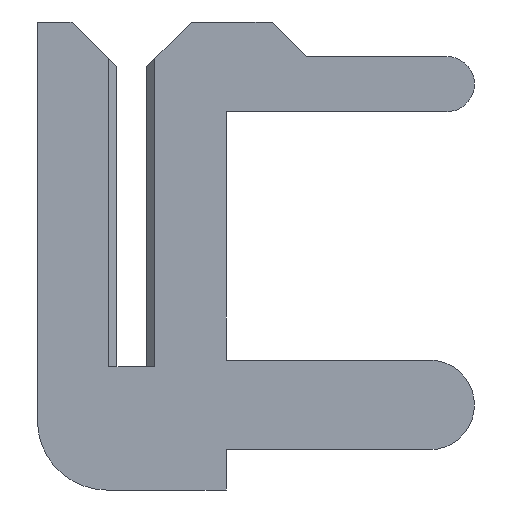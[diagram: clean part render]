
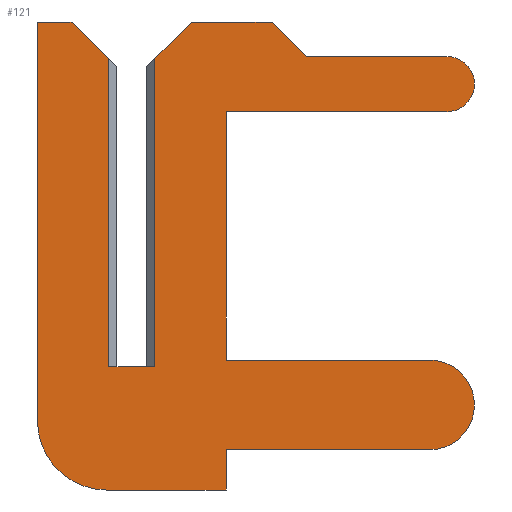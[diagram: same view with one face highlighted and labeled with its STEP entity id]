
A CAD part, left-side view. The second image highlights one B-rep face of the part: STEP entity #121.
In plain terms, the highlighted planar face has unit normal (-1, 0, 0).
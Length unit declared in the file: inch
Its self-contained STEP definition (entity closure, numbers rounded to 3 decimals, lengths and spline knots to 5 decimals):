
#1 = CARTESIAN_POINT ( 'NONE',  ( -0.01, -0.041, -0.0535 ) ) ;
#10 = CARTESIAN_POINT ( 'NONE',  ( -0.01, 0.041, -0.0235 ) ) ;
#18 = CARTESIAN_POINT ( 'NONE',  ( -0.01, 0.011, -0.0235 ) ) ;
#28 = ORIENTED_EDGE ( 'NONE', *, *, #631, .F. ) ;
#32 = DIRECTION ( 'NONE',  ( 0., 1., 0. ) ) ;
#33 = LINE ( 'NONE', #1293, #72 ) ;
#36 = VECTOR ( 'NONE', #32, 39.37008 ) ;
#49 = CIRCLE ( 'NONE', #253, 0.03 ) ;
#51 = AXIS2_PLACEMENT_3D ( 'NONE', #1385, #256, #1373 ) ;
#72 = VECTOR ( 'NONE', #274, 39.37008 ) ;
#87 = VERTEX_POINT ( 'NONE', #1380 ) ;
#98 = CARTESIAN_POINT ( 'NONE',  ( -0.01, -0.01, 0.134 ) ) ;
#117 = LINE ( 'NONE', #1328, #998 ) ;
#119 = ORIENTED_EDGE ( 'NONE', *, *, #770, .F. ) ;
#121 = ADVANCED_FACE ( 'NONE', ( #1006 ), #711, .T. ) ;
#137 = DIRECTION ( 'NONE',  ( 0., 0., 1. ) ) ;
#139 = VERTEX_POINT ( 'NONE', #268 ) ;
#145 = CARTESIAN_POINT ( 'NONE',  ( -0.01, -0.0065, 0.1305 ) ) ;
#150 = LINE ( 'NONE', #1226, #934 ) ;
#159 = EDGE_CURVE ( 'NONE', #396, #87, #238, .T. ) ;
#160 = CARTESIAN_POINT ( 'NONE',  ( -0.01, -0.01, 0.15 ) ) ;
#161 = LINE ( 'NONE', #1031, #1285 ) ;
#162 = VERTEX_POINT ( 'NONE', #1163 ) ;
#166 = CARTESIAN_POINT ( 'NONE',  ( -0.01, -0.041, -0.036 ) ) ;
#169 = DIRECTION ( 'NONE',  ( 0., 0., 1. ) ) ;
#177 = VERTEX_POINT ( 'NONE', #378 ) ;
#179 = ORIENTED_EDGE ( 'NONE', *, *, #1287, .F. ) ;
#181 = DIRECTION ( 'NONE',  ( 0., -0.707, 0.707 ) ) ;
#195 = VECTOR ( 'NONE', #435, 39.37008 ) ;
#196 = EDGE_CURVE ( 'NONE', #162, #177, #1047, .T. ) ;
#201 = CARTESIAN_POINT ( 'NONE',  ( -0.01, 0.026, 0.15 ) ) ;
#235 = VECTOR ( 'NONE', #595, 39.37008 ) ;
#238 = LINE ( 'NONE', #357, #1157 ) ;
#253 = AXIS2_PLACEMENT_3D ( 'NONE', #18, #1182, #1383 ) ;
#256 = DIRECTION ( 'NONE',  ( -1., 0., 0. ) ) ;
#268 = CARTESIAN_POINT ( 'NONE',  ( -0.01, -0.076, 0.135 ) ) ;
#271 = DIRECTION ( 'NONE',  ( 0., 0., -1. ) ) ;
#274 = DIRECTION ( 'NONE',  ( 0., -1., 0. ) ) ;
#292 = CIRCLE ( 'NONE', #353, 0.012 ) ;
#306 = DIRECTION ( 'NONE',  ( 0., 1., 0. ) ) ;
#334 = VERTEX_POINT ( 'NONE', #822 ) ;
#353 = AXIS2_PLACEMENT_3D ( 'NONE', #579, #693, #845 ) ;
#357 = CARTESIAN_POINT ( 'NONE',  ( -0.01, -0.041, 0.003 ) ) ;
#358 = LINE ( 'NONE', #496, #1228 ) ;
#360 = ORIENTED_EDGE ( 'NONE', *, *, #1177, .F. ) ;
#362 = VECTOR ( 'NONE', #696, 39.37008 ) ;
#377 = EDGE_CURVE ( 'NONE', #813, #678, #1231, .T. ) ;
#378 = CARTESIAN_POINT ( 'NONE',  ( -0.01, 0.01, 0.134 ) ) ;
#382 = DIRECTION ( 'NONE',  ( 0., 0., -1. ) ) ;
#385 = CARTESIAN_POINT ( 'NONE',  ( -0.01, -0.041, 0.111 ) ) ;
#388 = DIRECTION ( 'NONE',  ( 0., -1., 0. ) ) ;
#396 = VERTEX_POINT ( 'NONE', #385 ) ;
#403 = CARTESIAN_POINT ( 'NONE',  ( -0.01, -0.1295, -0.036 ) ) ;
#414 = EDGE_CURVE ( 'NONE', #1224, #334, #425, .T. ) ;
#420 = ORIENTED_EDGE ( 'NONE', *, *, #196, .T. ) ;
#425 = LINE ( 'NONE', #160, #1156 ) ;
#433 = DIRECTION ( 'NONE',  ( 0., 0., 1. ) ) ;
#435 = DIRECTION ( 'NONE',  ( 0., -1., 0. ) ) ;
#454 = ORIENTED_EDGE ( 'NONE', *, *, #689, .F. ) ;
#482 = VERTEX_POINT ( 'NONE', #1026 ) ;
#495 = VERTEX_POINT ( 'NONE', #574 ) ;
#496 = CARTESIAN_POINT ( 'NONE',  ( -0.01, 0.0065, 0.1305 ) ) ;
#500 = DIRECTION ( 'NONE',  ( 1., 0., 0. ) ) ;
#509 = VERTEX_POINT ( 'NONE', #1264 ) ;
#521 = ORIENTED_EDGE ( 'NONE', *, *, #715, .F. ) ;
#543 = DIRECTION ( 'NONE',  ( 0., -1., 0. ) ) ;
#559 = EDGE_CURVE ( 'NONE', #678, #561, #1175, .T. ) ;
#561 = VERTEX_POINT ( 'NONE', #1255 ) ;
#570 = ORIENTED_EDGE ( 'NONE', *, *, #414, .T. ) ;
#574 = CARTESIAN_POINT ( 'NONE',  ( -0.01, -0.026, 0.15 ) ) ;
#579 = CARTESIAN_POINT ( 'NONE',  ( -0.01, -0.137, 0.123 ) ) ;
#580 = VECTOR ( 'NONE', #137, 39.37008 ) ;
#595 = DIRECTION ( 'NONE',  ( 0., 1., 0. ) ) ;
#599 = ORIENTED_EDGE ( 'NONE', *, *, #1278, .F. ) ;
#623 = EDGE_LOOP ( 'NONE', ( #119, #570, #1122, #420, #521, #756, #599, #28, #823, #768, #660, #1046, #454, #803, #1327, #360, #1041, #179, #1098 ) ) ;
#631 = EDGE_CURVE ( 'NONE', #509, #1040, #49, .T. ) ;
#640 = VERTEX_POINT ( 'NONE', #801 ) ;
#642 = EDGE_CURVE ( 'NONE', #139, #721, #161, .T. ) ;
#645 = CARTESIAN_POINT ( 'NONE',  ( -0.01, 0.041, 0.15 ) ) ;
#651 = VERTEX_POINT ( 'NONE', #831 ) ;
#660 = ORIENTED_EDGE ( 'NONE', *, *, #377, .F. ) ;
#665 = EDGE_CURVE ( 'NONE', #1078, #396, #667, .T. ) ;
#667 = LINE ( 'NONE', #944, #235 ) ;
#678 = VERTEX_POINT ( 'NONE', #166 ) ;
#689 = EDGE_CURVE ( 'NONE', #87, #1140, #33, .T. ) ;
#692 = LINE ( 'NONE', #875, #195 ) ;
#693 = DIRECTION ( 'NONE',  ( 1., 0., 0. ) ) ;
#696 = DIRECTION ( 'NONE',  ( 0., 0., -1. ) ) ;
#705 = LINE ( 'NONE', #145, #868 ) ;
#711 = PLANE ( 'NONE',  #51 ) ;
#715 = EDGE_CURVE ( 'NONE', #651, #177, #358, .T. ) ;
#721 = VERTEX_POINT ( 'NONE', #955 ) ;
#745 = CIRCLE ( 'NONE', #1386, 0.0195 ) ;
#756 = ORIENTED_EDGE ( 'NONE', *, *, #1114, .F. ) ;
#768 = ORIENTED_EDGE ( 'NONE', *, *, #559, .F. ) ;
#770 = EDGE_CURVE ( 'NONE', #1224, #495, #705, .T. ) ;
#787 = EDGE_CURVE ( 'NONE', #561, #509, #848, .T. ) ;
#801 = CARTESIAN_POINT ( 'NONE',  ( -0.01, -0.061, 0.15 ) ) ;
#803 = ORIENTED_EDGE ( 'NONE', *, *, #159, .F. ) ;
#813 = VERTEX_POINT ( 'NONE', #403 ) ;
#822 = CARTESIAN_POINT ( 'NONE',  ( -0.01, -0.01, 0. ) ) ;
#823 = ORIENTED_EDGE ( 'NONE', *, *, #787, .F. ) ;
#831 = CARTESIAN_POINT ( 'NONE',  ( -0.01, 0.026, 0.15 ) ) ;
#837 = DIRECTION ( 'NONE',  ( 0., -0.707, -0.707 ) ) ;
#845 = DIRECTION ( 'NONE',  ( 0., 0., 1. ) ) ;
#848 = LINE ( 'NONE', #1190, #1409 ) ;
#868 = VECTOR ( 'NONE', #181, 39.37008 ) ;
#870 = EDGE_CURVE ( 'NONE', #1140, #813, #745, .T. ) ;
#875 = CARTESIAN_POINT ( 'NONE',  ( -0.01, 0.0065, 0. ) ) ;
#886 = DIRECTION ( 'NONE',  ( 0., -1., 0. ) ) ;
#934 = VECTOR ( 'NONE', #994, 39.37008 ) ;
#944 = CARTESIAN_POINT ( 'NONE',  ( -0.01, -0.041, 0.111 ) ) ;
#955 = CARTESIAN_POINT ( 'NONE',  ( -0.01, -0.137, 0.135 ) ) ;
#974 = CARTESIAN_POINT ( 'NONE',  ( -0.01, -0.137, 0.111 ) ) ;
#978 = EDGE_CURVE ( 'NONE', #495, #640, #117, .T. ) ;
#994 = DIRECTION ( 'NONE',  ( 0., -0.707, -0.707 ) ) ;
#998 = VECTOR ( 'NONE', #886, 39.37008 ) ;
#1006 = FACE_OUTER_BOUND ( 'NONE', #623, .T. ) ;
#1018 = EDGE_CURVE ( 'NONE', #162, #334, #692, .T. ) ;
#1026 = CARTESIAN_POINT ( 'NONE',  ( -0.01, 0.041, 0.15 ) ) ;
#1031 = CARTESIAN_POINT ( 'NONE',  ( -0.01, -0.137, 0.135 ) ) ;
#1040 = VERTEX_POINT ( 'NONE', #10 ) ;
#1041 = ORIENTED_EDGE ( 'NONE', *, *, #642, .F. ) ;
#1046 = ORIENTED_EDGE ( 'NONE', *, *, #870, .F. ) ;
#1047 = LINE ( 'NONE', #1051, #580 ) ;
#1051 = CARTESIAN_POINT ( 'NONE',  ( -0.01, 0.01, -0.0235 ) ) ;
#1078 = VERTEX_POINT ( 'NONE', #974 ) ;
#1096 = CARTESIAN_POINT ( 'NONE',  ( -0.01, -0.1295, 0.003 ) ) ;
#1098 = ORIENTED_EDGE ( 'NONE', *, *, #978, .F. ) ;
#1114 = EDGE_CURVE ( 'NONE', #482, #651, #1238, .T. ) ;
#1122 = ORIENTED_EDGE ( 'NONE', *, *, #1018, .F. ) ;
#1140 = VERTEX_POINT ( 'NONE', #1096 ) ;
#1156 = VECTOR ( 'NONE', #271, 39.37008 ) ;
#1157 = VECTOR ( 'NONE', #382, 39.37008 ) ;
#1163 = CARTESIAN_POINT ( 'NONE',  ( -0.01, 0.01, 0. ) ) ;
#1175 = LINE ( 'NONE', #1, #362 ) ;
#1177 = EDGE_CURVE ( 'NONE', #721, #1078, #292, .T. ) ;
#1182 = DIRECTION ( 'NONE',  ( 1., 0., 0. ) ) ;
#1186 = CARTESIAN_POINT ( 'NONE',  ( -0.01, -0.1295, -0.0165 ) ) ;
#1190 = CARTESIAN_POINT ( 'NONE',  ( -0.01, 0.011, -0.0535 ) ) ;
#1214 = VECTOR ( 'NONE', #543, 39.37008 ) ;
#1224 = VERTEX_POINT ( 'NONE', #98 ) ;
#1226 = CARTESIAN_POINT ( 'NONE',  ( -0.01, -0.076, 0.135 ) ) ;
#1228 = VECTOR ( 'NONE', #837, 39.37008 ) ;
#1231 = LINE ( 'NONE', #1295, #36 ) ;
#1238 = LINE ( 'NONE', #201, #1214 ) ;
#1254 = LINE ( 'NONE', #645, #1270 ) ;
#1255 = CARTESIAN_POINT ( 'NONE',  ( -0.01, -0.041, -0.0535 ) ) ;
#1264 = CARTESIAN_POINT ( 'NONE',  ( -0.01, 0.011, -0.0535 ) ) ;
#1270 = VECTOR ( 'NONE', #433, 39.37008 ) ;
#1278 = EDGE_CURVE ( 'NONE', #1040, #482, #1254, .T. ) ;
#1285 = VECTOR ( 'NONE', #388, 39.37008 ) ;
#1287 = EDGE_CURVE ( 'NONE', #640, #139, #150, .T. ) ;
#1293 = CARTESIAN_POINT ( 'NONE',  ( -0.01, -0.1295, 0.003 ) ) ;
#1295 = CARTESIAN_POINT ( 'NONE',  ( -0.01, -0.041, -0.036 ) ) ;
#1327 = ORIENTED_EDGE ( 'NONE', *, *, #665, .F. ) ;
#1328 = CARTESIAN_POINT ( 'NONE',  ( -0.01, -0.026, 0.15 ) ) ;
#1373 = DIRECTION ( 'NONE',  ( 0., 0., 1. ) ) ;
#1380 = CARTESIAN_POINT ( 'NONE',  ( -0.01, -0.041, 0.003 ) ) ;
#1383 = DIRECTION ( 'NONE',  ( 0., 0., 1. ) ) ;
#1385 = CARTESIAN_POINT ( 'NONE',  ( -0.01, 0.011, -0.0235 ) ) ;
#1386 = AXIS2_PLACEMENT_3D ( 'NONE', #1186, #500, #169 ) ;
#1409 = VECTOR ( 'NONE', #306, 39.37008 ) ;
